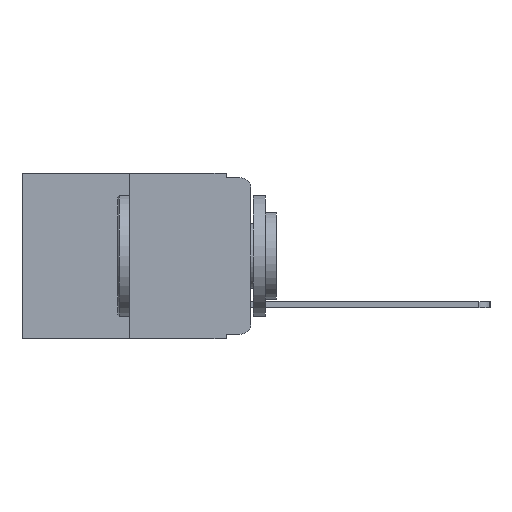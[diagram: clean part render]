
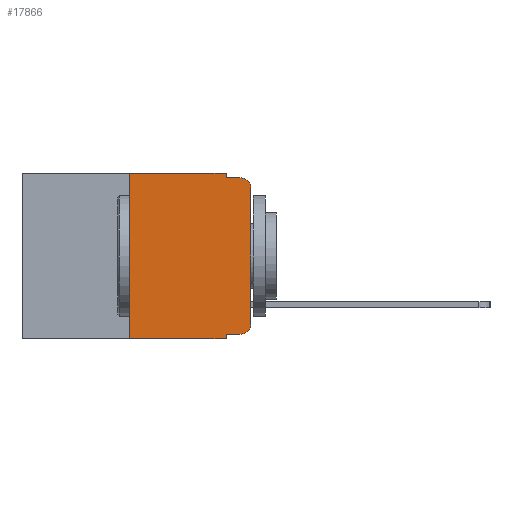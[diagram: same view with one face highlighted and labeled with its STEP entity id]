
A CAD part, left-side view. The second image highlights one B-rep face of the part: STEP entity #17866.
In plain terms, the highlighted planar face has unit normal (-1, 0, 0).
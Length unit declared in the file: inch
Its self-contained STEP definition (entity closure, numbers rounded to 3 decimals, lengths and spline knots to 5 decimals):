
#93 = EDGE_CURVE ( 'NONE', #4902, #10560, #13722, .T. ) ;
#456 = DIRECTION ( 'NONE',  ( 0., -1., 0. ) ) ;
#476 = CARTESIAN_POINT ( 'NONE',  ( 0., 0.051, 0. ) ) ;
#488 = CARTESIAN_POINT ( 'NONE',  ( 0., 0.051, -0.333 ) ) ;
#923 = VERTEX_POINT ( 'NONE', #16691 ) ;
#1089 = CARTESIAN_POINT ( 'NONE',  ( 0., 0.051, 0. ) ) ;
#1263 = EDGE_CURVE ( 'NONE', #7909, #14794, #4333, .T. ) ;
#2126 = AXIS2_PLACEMENT_3D ( 'NONE', #3371, #12064, #3452 ) ;
#2252 = CIRCLE ( 'NONE', #7239, 0.02 ) ;
#2317 = VECTOR ( 'NONE', #17432, 39.37008 ) ;
#2403 = EDGE_CURVE ( 'NONE', #10560, #923, #2252, .T. ) ;
#2544 = ORIENTED_EDGE ( 'NONE', *, *, #8932, .T. ) ;
#2547 = VERTEX_POINT ( 'NONE', #17686 ) ;
#3288 = VERTEX_POINT ( 'NONE', #3933 ) ;
#3371 = CARTESIAN_POINT ( 'NONE',  ( 0., 0.473, 0. ) ) ;
#3452 = DIRECTION ( 'NONE',  ( 0., 0., -1. ) ) ;
#3933 = CARTESIAN_POINT ( 'NONE',  ( 0., 0.051, -0.01 ) ) ;
#4333 = LINE ( 'NONE', #17716, #7850 ) ;
#4391 = LINE ( 'NONE', #14267, #11570 ) ;
#4902 = VERTEX_POINT ( 'NONE', #488 ) ;
#5354 = EDGE_LOOP ( 'NONE', ( #11054, #2544, #11106, #11393, #11415, #11437, #11661, #11714, #13399, #14199 ) ) ;
#6427 = EDGE_CURVE ( 'NONE', #2547, #9748, #4391, .T. ) ;
#6901 = CARTESIAN_POINT ( 'NONE',  ( 0., 0.051, -0.333 ) ) ;
#6953 = EDGE_CURVE ( 'NONE', #923, #8474, #10324, .T. ) ;
#7239 = AXIS2_PLACEMENT_3D ( 'NONE', #14944, #15009, #15107 ) ;
#7749 = CARTESIAN_POINT ( 'NONE',  ( 0., 0.051, 0. ) ) ;
#7850 = VECTOR ( 'NONE', #16908, 39.37008 ) ;
#7909 = VERTEX_POINT ( 'NONE', #16260 ) ;
#8069 = VECTOR ( 'NONE', #11871, 39.37008 ) ;
#8222 = CIRCLE ( 'NONE', #15992, 0.02 ) ;
#8363 = VECTOR ( 'NONE', #456, 39.37008 ) ;
#8474 = VERTEX_POINT ( 'NONE', #13889 ) ;
#8561 = LINE ( 'NONE', #7749, #8069 ) ;
#8932 = EDGE_CURVE ( 'NONE', #8474, #16600, #8222, .T. ) ;
#9257 = CARTESIAN_POINT ( 'NONE',  ( 0., 0., 0. ) ) ;
#9748 = VERTEX_POINT ( 'NONE', #1089 ) ;
#10242 = CARTESIAN_POINT ( 'NONE',  ( 0., 0.051, -0.343 ) ) ;
#10324 = LINE ( 'NONE', #9257, #2317 ) ;
#10560 = VERTEX_POINT ( 'NONE', #13741 ) ;
#10791 = EDGE_CURVE ( 'NONE', #3288, #16600, #12297, .T. ) ;
#11054 = ORIENTED_EDGE ( 'NONE', *, *, #6953, .T. ) ;
#11106 = ORIENTED_EDGE ( 'NONE', *, *, #10791, .F. ) ;
#11393 = ORIENTED_EDGE ( 'NONE', *, *, #11645, .F. ) ;
#11415 = ORIENTED_EDGE ( 'NONE', *, *, #6427, .F. ) ;
#11437 = ORIENTED_EDGE ( 'NONE', *, *, #12430, .F. ) ;
#11570 = VECTOR ( 'NONE', #11689, 39.37008 ) ;
#11645 = EDGE_CURVE ( 'NONE', #9748, #3288, #8561, .T. ) ;
#11661 = ORIENTED_EDGE ( 'NONE', *, *, #1263, .T. ) ;
#11689 = DIRECTION ( 'NONE',  ( 0., -1., 0. ) ) ;
#11712 = LINE ( 'NONE', #14449, #17754 ) ;
#11714 = ORIENTED_EDGE ( 'NONE', *, *, #17334, .F. ) ;
#11871 = DIRECTION ( 'NONE',  ( 0., 0., -1. ) ) ;
#12064 = DIRECTION ( 'NONE',  ( 1., 0., 0. ) ) ;
#12297 = LINE ( 'NONE', #13415, #8363 ) ;
#12430 = EDGE_CURVE ( 'NONE', #7909, #2547, #11712, .T. ) ;
#13111 = CARTESIAN_POINT ( 'NONE',  ( 0., 0.02, -0.01 ) ) ;
#13345 = VECTOR ( 'NONE', #14852, 39.37008 ) ;
#13399 = ORIENTED_EDGE ( 'NONE', *, *, #93, .T. ) ;
#13415 = CARTESIAN_POINT ( 'NONE',  ( 0., 0.051, -0.01 ) ) ;
#13722 = LINE ( 'NONE', #6901, #13345 ) ;
#13741 = CARTESIAN_POINT ( 'NONE',  ( 0., 0.02, -0.333 ) ) ;
#13889 = CARTESIAN_POINT ( 'NONE',  ( 0., 0., -0.03 ) ) ;
#14199 = ORIENTED_EDGE ( 'NONE', *, *, #2403, .T. ) ;
#14200 = VECTOR ( 'NONE', #14737, 39.37008 ) ;
#14267 = CARTESIAN_POINT ( 'NONE',  ( 0., 0.473, 0. ) ) ;
#14449 = CARTESIAN_POINT ( 'NONE',  ( 0., 0.25, 0. ) ) ;
#14602 = LINE ( 'NONE', #476, #14200 ) ;
#14737 = DIRECTION ( 'NONE',  ( 0., 0., -1. ) ) ;
#14794 = VERTEX_POINT ( 'NONE', #10242 ) ;
#14852 = DIRECTION ( 'NONE',  ( 0., -1., 0. ) ) ;
#14944 = CARTESIAN_POINT ( 'NONE',  ( 0., 0.02, -0.313 ) ) ;
#15009 = DIRECTION ( 'NONE',  ( -1., 0., 0. ) ) ;
#15107 = DIRECTION ( 'NONE',  ( 0., 0., -1. ) ) ;
#15560 = FACE_OUTER_BOUND ( 'NONE', #5354, .T. ) ;
#15662 = PLANE ( 'NONE',  #2126 ) ;
#15715 = DIRECTION ( 'NONE',  ( 0., 0., 1. ) ) ;
#15992 = AXIS2_PLACEMENT_3D ( 'NONE', #17651, #17639, #17622 ) ;
#16260 = CARTESIAN_POINT ( 'NONE',  ( 0., 0.25, -0.343 ) ) ;
#16600 = VERTEX_POINT ( 'NONE', #13111 ) ;
#16691 = CARTESIAN_POINT ( 'NONE',  ( 0., 0., -0.313 ) ) ;
#16908 = DIRECTION ( 'NONE',  ( 0., -1., 0. ) ) ;
#17334 = EDGE_CURVE ( 'NONE', #4902, #14794, #14602, .T. ) ;
#17432 = DIRECTION ( 'NONE',  ( 0., 0., 1. ) ) ;
#17622 = DIRECTION ( 'NONE',  ( 0., 0., -1. ) ) ;
#17639 = DIRECTION ( 'NONE',  ( -1., 0., 0. ) ) ;
#17651 = CARTESIAN_POINT ( 'NONE',  ( 0., 0.02, -0.03 ) ) ;
#17686 = CARTESIAN_POINT ( 'NONE',  ( 0., 0.25, 0. ) ) ;
#17716 = CARTESIAN_POINT ( 'NONE',  ( 0., 0.473, -0.343 ) ) ;
#17754 = VECTOR ( 'NONE', #15715, 39.37008 ) ;
#17866 = ADVANCED_FACE ( 'NONE', ( #15560 ), #15662, .F. ) ;
